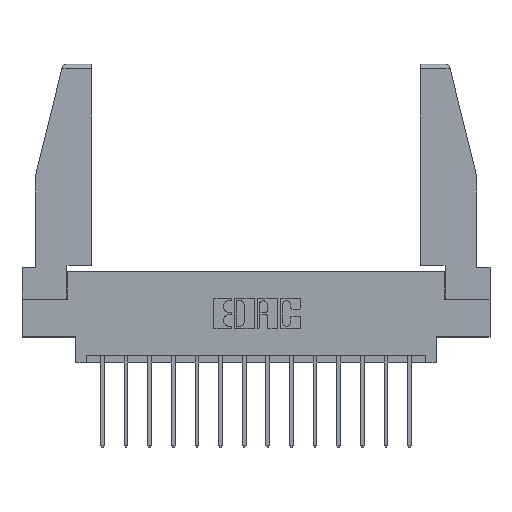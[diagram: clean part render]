
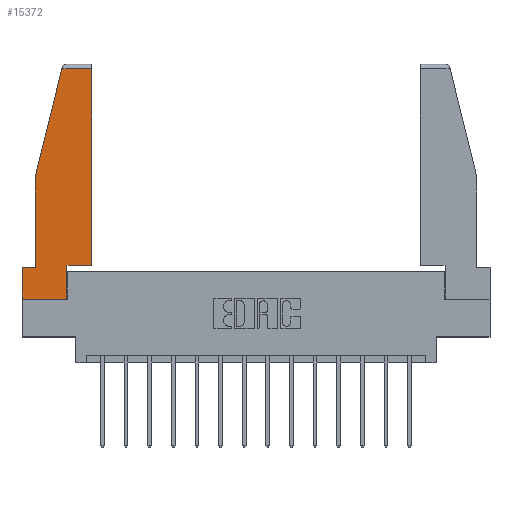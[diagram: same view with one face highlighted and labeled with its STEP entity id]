
A CAD part, top view. The second image highlights one B-rep face of the part: STEP entity #15372.
In plain terms, the highlighted planar face has unit normal (0, 0, 1).
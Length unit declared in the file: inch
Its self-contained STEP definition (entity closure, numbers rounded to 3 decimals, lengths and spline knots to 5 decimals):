
#438 = ORIENTED_EDGE ( 'NONE', *, *, #14922, .T. ) ;
#1914 = VERTEX_POINT ( 'NONE', #7091 ) ;
#2059 = ORIENTED_EDGE ( 'NONE', *, *, #14176, .T. ) ;
#2276 = ORIENTED_EDGE ( 'NONE', *, *, #5842, .T. ) ;
#2445 = DIRECTION ( 'NONE',  ( 0., 1., 0. ) ) ;
#2628 = CARTESIAN_POINT ( 'NONE',  ( 0., 0.21, 0. ) ) ;
#3080 = EDGE_CURVE ( 'NONE', #5032, #8658, #13461, .T. ) ;
#3359 = CARTESIAN_POINT ( 'NONE',  ( 0.086, 0.8, 0. ) ) ;
#3445 = VECTOR ( 'NONE', #2445, 39.37008 ) ;
#3542 = VERTEX_POINT ( 'NONE', #8998 ) ;
#3666 = VECTOR ( 'NONE', #4002, 39.37008 ) ;
#3835 = CARTESIAN_POINT ( 'NONE',  ( 0., 0.21, 0. ) ) ;
#3893 = ORIENTED_EDGE ( 'NONE', *, *, #5023, .T. ) ;
#3938 = CARTESIAN_POINT ( 'NONE',  ( 0., 1.52, 0. ) ) ;
#4002 = DIRECTION ( 'NONE',  ( -1., 0., 0. ) ) ;
#4507 = DIRECTION ( 'NONE',  ( 1., 0., 0. ) ) ;
#4607 = VERTEX_POINT ( 'NONE', #14067 ) ;
#4704 = CARTESIAN_POINT ( 'NONE',  ( 0.297, 0.223, 0. ) ) ;
#4804 = PLANE ( 'NONE',  #7811 ) ;
#4916 = ORIENTED_EDGE ( 'NONE', *, *, #13222, .T. ) ;
#5023 = EDGE_CURVE ( 'NONE', #4607, #5380, #14395, .T. ) ;
#5032 = VERTEX_POINT ( 'NONE', #2628 ) ;
#5066 = VECTOR ( 'NONE', #15804, 39.37008 ) ;
#5380 = VERTEX_POINT ( 'NONE', #11152 ) ;
#5385 = DIRECTION ( 'NONE',  ( 0., -1., 0. ) ) ;
#5412 = VECTOR ( 'NONE', #13139, 39.37008 ) ;
#5473 = VERTEX_POINT ( 'NONE', #3359 ) ;
#5666 = LINE ( 'NONE', #3835, #5066 ) ;
#5842 = EDGE_CURVE ( 'NONE', #1914, #15104, #7638, .T. ) ;
#6640 = DIRECTION ( 'NONE',  ( 0., -1., 0. ) ) ;
#6972 = CARTESIAN_POINT ( 'NONE',  ( 0., 0., 0. ) ) ;
#7091 = CARTESIAN_POINT ( 'NONE',  ( 0.297, 0., 0. ) ) ;
#7479 = FACE_OUTER_BOUND ( 'NONE', #8470, .T. ) ;
#7522 = LINE ( 'NONE', #11900, #5412 ) ;
#7638 = LINE ( 'NONE', #17075, #3445 ) ;
#7811 = AXIS2_PLACEMENT_3D ( 'NONE', #15177, #13835, #11284 ) ;
#8014 = ORIENTED_EDGE ( 'NONE', *, *, #10169, .T. ) ;
#8470 = EDGE_LOOP ( 'NONE', ( #16337, #3893, #438, #12812, #4916, #12700, #8014, #2276, #2059 ) ) ;
#8561 = VECTOR ( 'NONE', #6640, 39.37008 ) ;
#8658 = VERTEX_POINT ( 'NONE', #17077 ) ;
#8704 = LINE ( 'NONE', #6972, #13406 ) ;
#8766 = LINE ( 'NONE', #13395, #9998 ) ;
#8978 = VERTEX_POINT ( 'NONE', #13971 ) ;
#8998 = CARTESIAN_POINT ( 'NONE',  ( 0.086, 0.21, 0. ) ) ;
#9530 = DIRECTION ( 'NONE',  ( -0.239, -0.971, 0. ) ) ;
#9998 = VECTOR ( 'NONE', #5385, 39.37008 ) ;
#10169 = EDGE_CURVE ( 'NONE', #8658, #1914, #8704, .T. ) ;
#11152 = CARTESIAN_POINT ( 'NONE',  ( 0.2636, 1.52, 0. ) ) ;
#11194 = VECTOR ( 'NONE', #9530, 39.37008 ) ;
#11284 = DIRECTION ( 'NONE',  ( 1., 0., 0. ) ) ;
#11900 = CARTESIAN_POINT ( 'NONE',  ( 0.297, 0.223, 0. ) ) ;
#12276 = EDGE_CURVE ( 'NONE', #8978, #4607, #12521, .T. ) ;
#12521 = LINE ( 'NONE', #16055, #16817 ) ;
#12700 = ORIENTED_EDGE ( 'NONE', *, *, #3080, .T. ) ;
#12812 = ORIENTED_EDGE ( 'NONE', *, *, #14015, .T. ) ;
#13139 = DIRECTION ( 'NONE',  ( 1., 0., 0. ) ) ;
#13222 = EDGE_CURVE ( 'NONE', #3542, #5032, #5666, .T. ) ;
#13395 = CARTESIAN_POINT ( 'NONE',  ( 0.086, 0.8, 0. ) ) ;
#13406 = VECTOR ( 'NONE', #4507, 39.37008 ) ;
#13461 = LINE ( 'NONE', #14991, #8561 ) ;
#13472 = CARTESIAN_POINT ( 'NONE',  ( 0.271, 1.55, 0. ) ) ;
#13619 = DIRECTION ( 'NONE',  ( 0., 1., 0. ) ) ;
#13835 = DIRECTION ( 'NONE',  ( 0., 0., 1. ) ) ;
#13971 = CARTESIAN_POINT ( 'NONE',  ( 0.461, 0.223, 0. ) ) ;
#14015 = EDGE_CURVE ( 'NONE', #5473, #3542, #8766, .T. ) ;
#14067 = CARTESIAN_POINT ( 'NONE',  ( 0.461, 1.52, 0. ) ) ;
#14176 = EDGE_CURVE ( 'NONE', #15104, #8978, #7522, .T. ) ;
#14395 = LINE ( 'NONE', #3938, #3666 ) ;
#14638 = LINE ( 'NONE', #13472, #11194 ) ;
#14922 = EDGE_CURVE ( 'NONE', #5380, #5473, #14638, .T. ) ;
#14991 = CARTESIAN_POINT ( 'NONE',  ( 0., 0.21, 0. ) ) ;
#15104 = VERTEX_POINT ( 'NONE', #4704 ) ;
#15177 = CARTESIAN_POINT ( 'NONE',  ( 0., 0., 0. ) ) ;
#15372 = ADVANCED_FACE ( 'NONE', ( #7479 ), #4804, .T. ) ;
#15804 = DIRECTION ( 'NONE',  ( -1., 0., 0. ) ) ;
#16055 = CARTESIAN_POINT ( 'NONE',  ( 0.461, 0.223, 0. ) ) ;
#16337 = ORIENTED_EDGE ( 'NONE', *, *, #12276, .T. ) ;
#16817 = VECTOR ( 'NONE', #13619, 39.37008 ) ;
#17075 = CARTESIAN_POINT ( 'NONE',  ( 0.297, 0., 0. ) ) ;
#17077 = CARTESIAN_POINT ( 'NONE',  ( 0., 0., 0. ) ) ;
